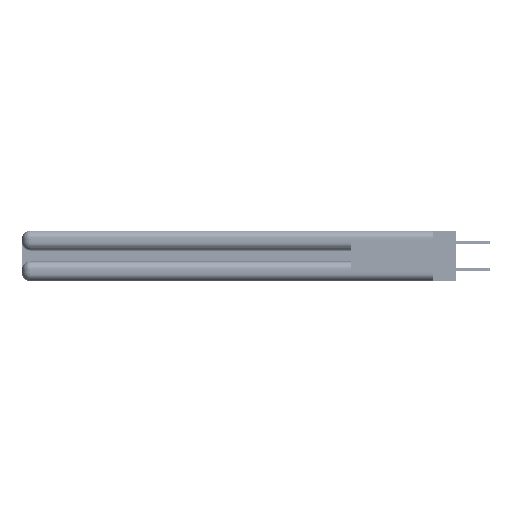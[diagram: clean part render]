
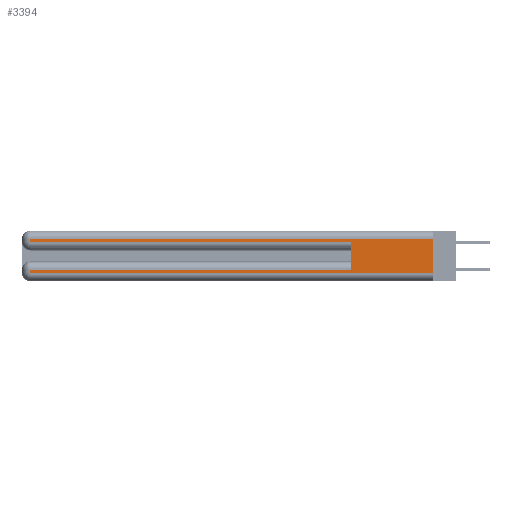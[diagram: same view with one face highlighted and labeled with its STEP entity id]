
A CAD part, left-side view. The second image highlights one B-rep face of the part: STEP entity #3394.
In plain terms, the highlighted planar face has unit normal (-1, 0, 0).
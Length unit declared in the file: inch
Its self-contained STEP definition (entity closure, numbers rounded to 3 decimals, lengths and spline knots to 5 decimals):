
#815 = CARTESIAN_POINT ( 'NONE',  ( 0., 2.94, 0.085 ) ) ;
#3293 = DIRECTION ( 'NONE',  ( 0., 1., 0. ) ) ;
#3375 = EDGE_CURVE ( 'NONE', #33151, #47616, #14041, .T. ) ;
#3394 = ADVANCED_FACE ( 'NONE', ( #30470 ), #34134, .F. ) ;
#3977 = CARTESIAN_POINT ( 'NONE',  ( 0., 2.94, 0.06 ) ) ;
#4473 = VERTEX_POINT ( 'NONE', #24808 ) ;
#5202 = ORIENTED_EDGE ( 'NONE', *, *, #27732, .T. ) ;
#5434 = CARTESIAN_POINT ( 'NONE',  ( 0., 0., 0.37 ) ) ;
#6640 = EDGE_CURVE ( 'NONE', #23116, #9244, #44030, .T. ) ;
#7373 = CARTESIAN_POINT ( 'NONE',  ( 0., 0., 0.085 ) ) ;
#7882 = CARTESIAN_POINT ( 'NONE',  ( 0., 0., 0.06 ) ) ;
#8437 = DIRECTION ( 'NONE',  ( 0., 0., -1. ) ) ;
#8764 = LINE ( 'NONE', #7373, #37983 ) ;
#9244 = VERTEX_POINT ( 'NONE', #31525 ) ;
#9523 = LINE ( 'NONE', #15679, #20328 ) ;
#10066 = VERTEX_POINT ( 'NONE', #41375 ) ;
#10827 = CARTESIAN_POINT ( 'NONE',  ( 0., 0., 0.37 ) ) ;
#11738 = CARTESIAN_POINT ( 'NONE',  ( 0., 0.6, 0.085 ) ) ;
#12159 = CARTESIAN_POINT ( 'NONE',  ( 0., 0., 0.31 ) ) ;
#13143 = VECTOR ( 'NONE', #44065, 39.37008 ) ;
#14041 = LINE ( 'NONE', #42140, #52060 ) ;
#14616 = AXIS2_PLACEMENT_3D ( 'NONE', #5434, #46364, #50616 ) ;
#15679 = CARTESIAN_POINT ( 'NONE',  ( 0., 0.6, 0.145 ) ) ;
#17586 = EDGE_CURVE ( 'NONE', #23116, #4473, #22842, .T. ) ;
#18200 = DIRECTION ( 'NONE',  ( 0., 0., -1. ) ) ;
#19084 = ORIENTED_EDGE ( 'NONE', *, *, #17586, .T. ) ;
#19229 = DIRECTION ( 'NONE',  ( 0., 0., 1. ) ) ;
#19806 = DIRECTION ( 'NONE',  ( 0., 1., 0. ) ) ;
#20328 = VECTOR ( 'NONE', #19229, 39.37008 ) ;
#22581 = DIRECTION ( 'NONE',  ( 0., 0., -1. ) ) ;
#22774 = VECTOR ( 'NONE', #43385, 39.37008 ) ;
#22842 = LINE ( 'NONE', #12159, #40629 ) ;
#23116 = VERTEX_POINT ( 'NONE', #30593 ) ;
#23943 = LINE ( 'NONE', #7882, #13143 ) ;
#24808 = CARTESIAN_POINT ( 'NONE',  ( 0., 2.94, 0.31 ) ) ;
#24969 = ORIENTED_EDGE ( 'NONE', *, *, #33427, .T. ) ;
#26247 = VECTOR ( 'NONE', #8437, 39.37008 ) ;
#27087 = ORIENTED_EDGE ( 'NONE', *, *, #41610, .F. ) ;
#27732 = EDGE_CURVE ( 'NONE', #10066, #45715, #48762, .T. ) ;
#27739 = EDGE_CURVE ( 'NONE', #48477, #33151, #8764, .T. ) ;
#28126 = VECTOR ( 'NONE', #22581, 39.37008 ) ;
#29826 = CARTESIAN_POINT ( 'NONE',  ( 0., 0.6, 0.285 ) ) ;
#30470 = FACE_OUTER_BOUND ( 'NONE', #33423, .T. ) ;
#30593 = CARTESIAN_POINT ( 'NONE',  ( 0., 0., 0.31 ) ) ;
#31525 = CARTESIAN_POINT ( 'NONE',  ( 0., 0., 0.06 ) ) ;
#33151 = VERTEX_POINT ( 'NONE', #815 ) ;
#33423 = EDGE_LOOP ( 'NONE', ( #49142, #19084, #46983, #5202, #27087, #34222, #46813, #24969 ) ) ;
#33427 = EDGE_CURVE ( 'NONE', #47616, #9244, #23943, .T. ) ;
#34134 = PLANE ( 'NONE',  #14616 ) ;
#34222 = ORIENTED_EDGE ( 'NONE', *, *, #27739, .T. ) ;
#36276 = CARTESIAN_POINT ( 'NONE',  ( 0., 2.94, 0.37 ) ) ;
#37983 = VECTOR ( 'NONE', #3293, 39.37008 ) ;
#39358 = EDGE_CURVE ( 'NONE', #4473, #10066, #46547, .T. ) ;
#40629 = VECTOR ( 'NONE', #19806, 39.37008 ) ;
#41375 = CARTESIAN_POINT ( 'NONE',  ( 0., 2.94, 0.285 ) ) ;
#41610 = EDGE_CURVE ( 'NONE', #48477, #45715, #9523, .T. ) ;
#42140 = CARTESIAN_POINT ( 'NONE',  ( 0., 2.94, 0.37 ) ) ;
#43385 = DIRECTION ( 'NONE',  ( 0., -1., 0. ) ) ;
#44030 = LINE ( 'NONE', #10827, #28126 ) ;
#44065 = DIRECTION ( 'NONE',  ( 0., -1., 0. ) ) ;
#45715 = VERTEX_POINT ( 'NONE', #29826 ) ;
#46364 = DIRECTION ( 'NONE',  ( 1., 0., 0. ) ) ;
#46547 = LINE ( 'NONE', #36276, #26247 ) ;
#46813 = ORIENTED_EDGE ( 'NONE', *, *, #3375, .T. ) ;
#46983 = ORIENTED_EDGE ( 'NONE', *, *, #39358, .T. ) ;
#47616 = VERTEX_POINT ( 'NONE', #3977 ) ;
#48477 = VERTEX_POINT ( 'NONE', #11738 ) ;
#48762 = LINE ( 'NONE', #51686, #22774 ) ;
#49142 = ORIENTED_EDGE ( 'NONE', *, *, #6640, .F. ) ;
#50616 = DIRECTION ( 'NONE',  ( 0., 0., -1. ) ) ;
#51686 = CARTESIAN_POINT ( 'NONE',  ( 0., 0., 0.285 ) ) ;
#52060 = VECTOR ( 'NONE', #18200, 39.37008 ) ;
